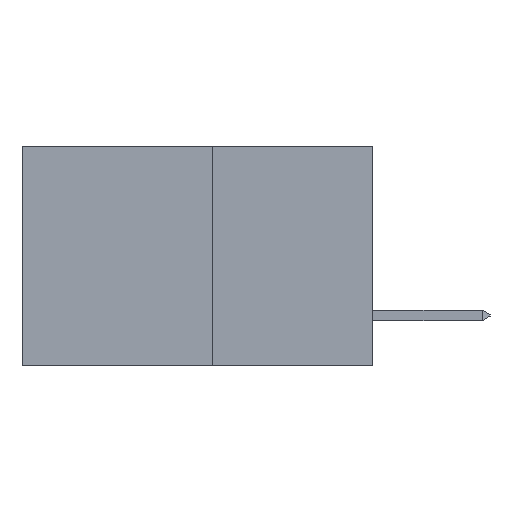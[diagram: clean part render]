
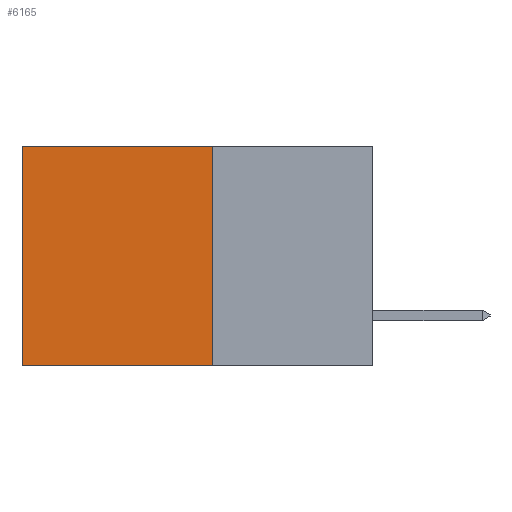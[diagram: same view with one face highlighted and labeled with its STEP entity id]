
A CAD part, left-side view. The second image highlights one B-rep face of the part: STEP entity #6165.
In plain terms, the highlighted planar face has unit normal (-1, 0, 0).
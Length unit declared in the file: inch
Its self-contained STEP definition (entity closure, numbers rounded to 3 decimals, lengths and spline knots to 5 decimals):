
#259 = DIRECTION ( 'NONE',  ( 0., 0., -1. ) ) ;
#609 = EDGE_LOOP ( 'NONE', ( #1635, #1150, #2134, #8710 ) ) ;
#789 = CARTESIAN_POINT ( 'NONE',  ( 0.277, 0.59, -0.37 ) ) ;
#1150 = ORIENTED_EDGE ( 'NONE', *, *, #5695, .F. ) ;
#1206 = DIRECTION ( 'NONE',  ( 1., 0., 0. ) ) ;
#1299 = CARTESIAN_POINT ( 'NONE',  ( 0.277, 0.27, -0.37 ) ) ;
#1382 = CARTESIAN_POINT ( 'NONE',  ( 0.277, 0.27, -0.37 ) ) ;
#1628 = LINE ( 'NONE', #8316, #3654 ) ;
#1635 = ORIENTED_EDGE ( 'NONE', *, *, #7241, .T. ) ;
#1848 = CARTESIAN_POINT ( 'NONE',  ( 0.277, 0.59, -0.37 ) ) ;
#1914 = AXIS2_PLACEMENT_3D ( 'NONE', #7790, #1206, #6391 ) ;
#2134 = ORIENTED_EDGE ( 'NONE', *, *, #8042, .F. ) ;
#2619 = LINE ( 'NONE', #1848, #4809 ) ;
#2635 = VECTOR ( 'NONE', #7246, 39.37008 ) ;
#3279 = DIRECTION ( 'NONE',  ( 0., 1., 0. ) ) ;
#3654 = VECTOR ( 'NONE', #3279, 39.37008 ) ;
#4809 = VECTOR ( 'NONE', #259, 39.37008 ) ;
#4826 = LINE ( 'NONE', #1382, #2635 ) ;
#5645 = PLANE ( 'NONE',  #1914 ) ;
#5652 = CARTESIAN_POINT ( 'NONE',  ( 0.277, 0.27, -0.37 ) ) ;
#5695 = EDGE_CURVE ( 'NONE', #9243, #7004, #4826, .T. ) ;
#6165 = ADVANCED_FACE ( 'NONE', ( #8397 ), #5645, .F. ) ;
#6391 = DIRECTION ( 'NONE',  ( 0., 0., -1. ) ) ;
#6397 = DIRECTION ( 'NONE',  ( 0., 0., -1. ) ) ;
#7004 = VERTEX_POINT ( 'NONE', #789 ) ;
#7119 = VECTOR ( 'NONE', #6397, 39.37008 ) ;
#7241 = EDGE_CURVE ( 'NONE', #9474, #7004, #2619, .T. ) ;
#7246 = DIRECTION ( 'NONE',  ( 0., 1., 0. ) ) ;
#7786 = CARTESIAN_POINT ( 'NONE',  ( 0.277, 0.27, 0. ) ) ;
#7790 = CARTESIAN_POINT ( 'NONE',  ( 0.277, 0.27, -0.37 ) ) ;
#7795 = EDGE_CURVE ( 'NONE', #8676, #9474, #1628, .T. ) ;
#8042 = EDGE_CURVE ( 'NONE', #8676, #9243, #8793, .T. ) ;
#8123 = CARTESIAN_POINT ( 'NONE',  ( 0.277, 0.59, 0. ) ) ;
#8316 = CARTESIAN_POINT ( 'NONE',  ( 0.277, 0.27, 0. ) ) ;
#8397 = FACE_OUTER_BOUND ( 'NONE', #609, .T. ) ;
#8676 = VERTEX_POINT ( 'NONE', #7786 ) ;
#8710 = ORIENTED_EDGE ( 'NONE', *, *, #7795, .T. ) ;
#8793 = LINE ( 'NONE', #5652, #7119 ) ;
#9243 = VERTEX_POINT ( 'NONE', #1299 ) ;
#9474 = VERTEX_POINT ( 'NONE', #8123 ) ;
